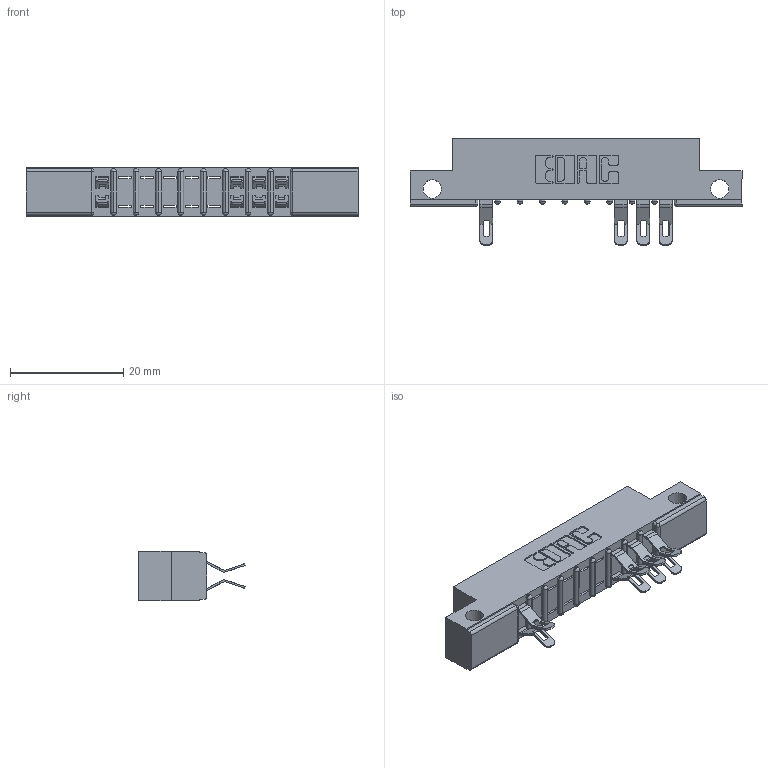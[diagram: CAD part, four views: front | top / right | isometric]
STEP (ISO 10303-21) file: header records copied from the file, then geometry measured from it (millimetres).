
FILE_DESCRIPTION (( 'STEP AP203' ), '1' );
FILE_NAME ('357-018-555-212.STEP', '2018-08-08T05:44:00', ( '' ), ( '' ), 'SwSTEP 2.0', 'SolidWorks 2016', '' );
FILE_SCHEMA (( 'CONFIG_CONTROL_DESIGN' ));
Length unit declared in the file: inch
Products named in the file (3): 307 Part_.128 Dia Side Mounting Holes; 307-290-001_555; 357-018-555-212
Assembly tree (9 placements, depth 2):
  357-018-555-212
    307 Part_.128 Dia Side Mounting Holes
    307-290-001_555  x8
Bounding box: 58.67 x 18.75 x 8.71 mm (x, y, z)
Volume: 3657.8 mm3; surface area: 5011.4 mm2
Topology: 9 solids, 9 shells, 716 faces, 2091 edges, 1354 vertices
Faces by surface type: plane 402, cylinder 294, sphere 20
Entity records: 12291 total; most frequent: CARTESIAN_POINT 2067, ORIENTED_EDGE 2056, DIRECTION 2036, EDGE_CURVE 1028, VECTOR 762, LINE 762, VERTEX_POINT 668, AXIS2_PLACEMENT_3D 637
